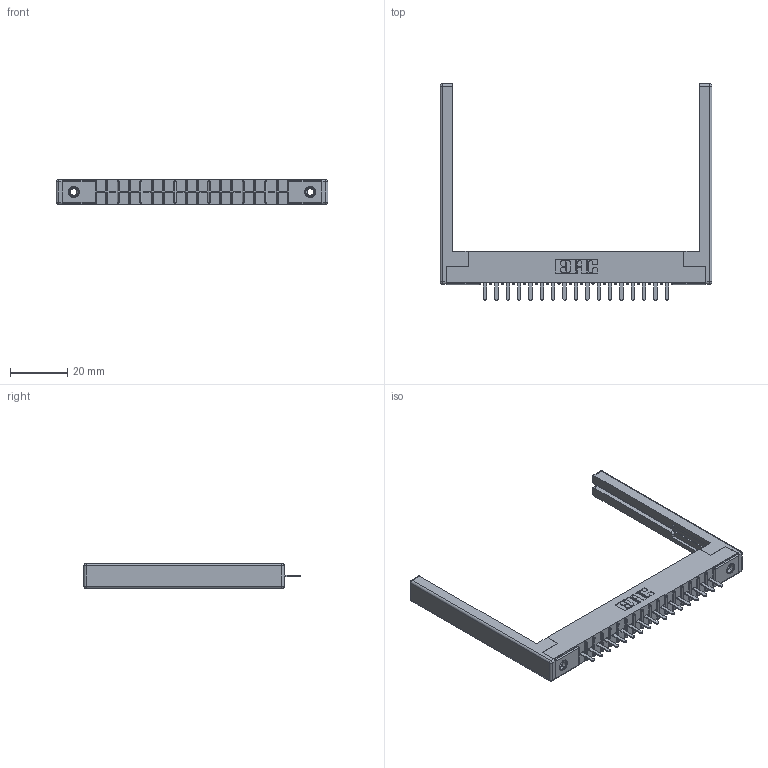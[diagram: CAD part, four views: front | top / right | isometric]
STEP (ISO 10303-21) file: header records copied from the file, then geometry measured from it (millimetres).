
FILE_DESCRIPTION (( 'STEP AP203' ), '1' );
FILE_NAME ('316-017-420-168.STEP', '2020-09-22T18:16:36', ( '' ), ( '' ), 'SwSTEP 2.0', 'SolidWorks 2020', '' );
FILE_SCHEMA (( 'CONFIG_CONTROL_DESIGN' ));
Length unit declared in the file: inch
Products named in the file (5): 316-017-420-168; 345-250-001_345-250-001-102; 306 Part_.156 Dia; 307-220-068; 306-290-001_120
Assembly tree (22 placements, depth 2):
  316-017-420-168
    306 Part_.156 Dia
    306-290-001_120  x17
    345-250-001_345-250-001-102  x2
    307-220-068  x2
Bounding box: 94.79 x 75.41 x 8.71 mm (x, y, z)
Volume: 11015.8 mm3; surface area: 13509.8 mm2
Topology: 22 solids, 22 shells, 1460 faces, 4055 edges, 2590 vertices
Faces by surface type: plane 955, cylinder 413, sphere 76, cone 12, torus 4
Entity records: 21807 total; most frequent: CARTESIAN_POINT 3623, DIRECTION 3588, ORIENTED_EDGE 3580, EDGE_CURVE 1790, LINE 1382, VECTOR 1382, VERTEX_POINT 1138, AXIS2_PLACEMENT_3D 1103
